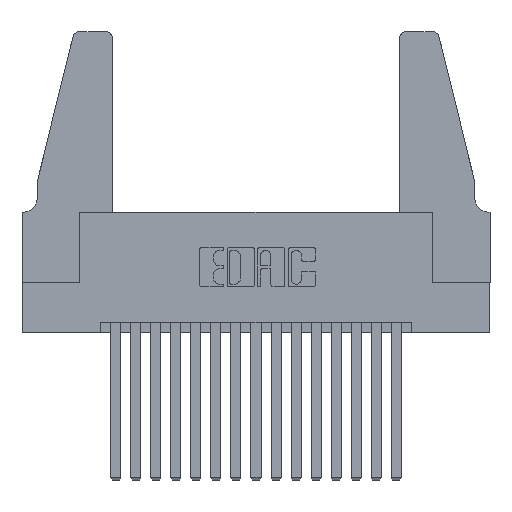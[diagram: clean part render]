
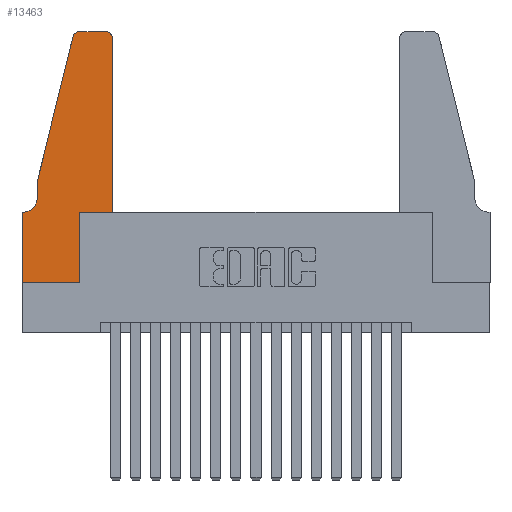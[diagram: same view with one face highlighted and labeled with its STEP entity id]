
A CAD part, top view. The second image highlights one B-rep face of the part: STEP entity #13463.
In plain terms, the highlighted planar face has unit normal (0, 0, 1).
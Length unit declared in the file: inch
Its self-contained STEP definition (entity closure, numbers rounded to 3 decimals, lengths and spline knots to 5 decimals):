
#137 = CARTESIAN_POINT ( 'NONE',  ( 0.284, 1.22, 0.37 ) ) ;
#166 = ORIENTED_EDGE ( 'NONE', *, *, #4814, .T. ) ;
#209 = LINE ( 'NONE', #13589, #14076 ) ;
#366 = DIRECTION ( 'NONE',  ( 0., 0., -1. ) ) ;
#385 = ORIENTED_EDGE ( 'NONE', *, *, #17398, .T. ) ;
#788 = CIRCLE ( 'NONE', #13161, 0.07 ) ;
#1159 = VECTOR ( 'NONE', #3147, 39.37008 ) ;
#1178 = EDGE_CURVE ( 'NONE', #5568, #14867, #12893, .T. ) ;
#1228 = EDGE_CURVE ( 'NONE', #10429, #8796, #16892, .T. ) ;
#1312 = EDGE_CURVE ( 'NONE', #3085, #3375, #16051, .T. ) ;
#1481 = DIRECTION ( 'NONE',  ( 1., 0., 0. ) ) ;
#1575 = DIRECTION ( 'NONE',  ( 0., 0., 1. ) ) ;
#1823 = DIRECTION ( 'NONE',  ( 0., 1., 0. ) ) ;
#1984 = CARTESIAN_POINT ( 'NONE',  ( 0.4205, 1.25, 0.37 ) ) ;
#2202 = CARTESIAN_POINT ( 'NONE',  ( 0.0755, 0.42, 0.37 ) ) ;
#2214 = LINE ( 'NONE', #5744, #1159 ) ;
#2564 = ORIENTED_EDGE ( 'NONE', *, *, #1178, .T. ) ;
#3085 = VERTEX_POINT ( 'NONE', #8862 ) ;
#3147 = DIRECTION ( 'NONE',  ( 1., 0., 0. ) ) ;
#3240 = CARTESIAN_POINT ( 'NONE',  ( 0.2605, 1.25, 0.37 ) ) ;
#3375 = VERTEX_POINT ( 'NONE', #8194 ) ;
#3391 = EDGE_CURVE ( 'NONE', #10705, #13900, #209, .T. ) ;
#3474 = CARTESIAN_POINT ( 'NONE',  ( 0.2865, 0.35, 0.37 ) ) ;
#3906 = CARTESIAN_POINT ( 'NONE',  ( 0.0055, 0.42, 0.37 ) ) ;
#3923 = FACE_OUTER_BOUND ( 'NONE', #4891, .T. ) ;
#3956 = LINE ( 'NONE', #12894, #6268 ) ;
#4252 = CARTESIAN_POINT ( 'NONE',  ( 0.4505, 0.35, 0.37 ) ) ;
#4470 = PLANE ( 'NONE',  #17057 ) ;
#4814 = EDGE_CURVE ( 'NONE', #3375, #9165, #5978, .T. ) ;
#4873 = VECTOR ( 'NONE', #11289, 39.37008 ) ;
#4891 = EDGE_LOOP ( 'NONE', ( #16648, #14484, #16259, #6245, #11322, #14737, #166, #10892, #2564, #385, #16778, #10352 ) ) ;
#5568 = VERTEX_POINT ( 'NONE', #9376 ) ;
#5744 = CARTESIAN_POINT ( 'NONE',  ( 0.4505, 0.35, 0.37 ) ) ;
#5761 = CARTESIAN_POINT ( 'NONE',  ( 0.4205, 1.22, 0.37 ) ) ;
#5942 = DIRECTION ( 'NONE',  ( -1., 0., 0. ) ) ;
#5945 = CARTESIAN_POINT ( 'NONE',  ( 0., 0., 0.37 ) ) ;
#5965 = VECTOR ( 'NONE', #1823, 39.37008 ) ;
#5978 = LINE ( 'NONE', #9507, #14577 ) ;
#6245 = ORIENTED_EDGE ( 'NONE', *, *, #8325, .T. ) ;
#6268 = VECTOR ( 'NONE', #16893, 39.37008 ) ;
#6347 = LINE ( 'NONE', #5945, #4873 ) ;
#6402 = CARTESIAN_POINT ( 'NONE',  ( 0.0755, 0.35, 0.37 ) ) ;
#6972 = EDGE_CURVE ( 'NONE', #10090, #10808, #15559, .T. ) ;
#7097 = CIRCLE ( 'NONE', #11618, 0.03 ) ;
#7509 = CARTESIAN_POINT ( 'NONE',  ( 0., 0., 0.37 ) ) ;
#7788 = CIRCLE ( 'NONE', #16339, 0.03 ) ;
#8117 = EDGE_CURVE ( 'NONE', #8409, #3085, #788, .T. ) ;
#8194 = CARTESIAN_POINT ( 'NONE',  ( 0., 0.35, 0.37 ) ) ;
#8314 = DIRECTION ( 'NONE',  ( 0., -1., 0. ) ) ;
#8325 = EDGE_CURVE ( 'NONE', #13900, #8409, #3956, .T. ) ;
#8409 = VERTEX_POINT ( 'NONE', #2202 ) ;
#8594 = DIRECTION ( 'NONE',  ( 0., 0., 1. ) ) ;
#8648 = CARTESIAN_POINT ( 'NONE',  ( 0., 0.35, 0.37 ) ) ;
#8796 = VERTEX_POINT ( 'NONE', #14611 ) ;
#8862 = CARTESIAN_POINT ( 'NONE',  ( 0.0055, 0.35, 0.37 ) ) ;
#9165 = VERTEX_POINT ( 'NONE', #7509 ) ;
#9376 = CARTESIAN_POINT ( 'NONE',  ( 0.2865, 0., 0.37 ) ) ;
#9507 = CARTESIAN_POINT ( 'NONE',  ( 0., 0., 0.37 ) ) ;
#9562 = DIRECTION ( 'NONE',  ( 0., 0., 1. ) ) ;
#10090 = VERTEX_POINT ( 'NONE', #13851 ) ;
#10174 = DIRECTION ( 'NONE',  ( -1., 0., 0. ) ) ;
#10352 = ORIENTED_EDGE ( 'NONE', *, *, #16832, .T. ) ;
#10429 = VERTEX_POINT ( 'NONE', #1984 ) ;
#10705 = VERTEX_POINT ( 'NONE', #12749 ) ;
#10747 = EDGE_CURVE ( 'NONE', #9165, #5568, #6347, .T. ) ;
#10808 = VERTEX_POINT ( 'NONE', #12856 ) ;
#10892 = ORIENTED_EDGE ( 'NONE', *, *, #10747, .T. ) ;
#10975 = DIRECTION ( 'NONE',  ( 1., 0., 0. ) ) ;
#11079 = CARTESIAN_POINT ( 'NONE',  ( 0.0755, 0.5, 0.37 ) ) ;
#11146 = VECTOR ( 'NONE', #16391, 39.37008 ) ;
#11289 = DIRECTION ( 'NONE',  ( 1., 0., 0. ) ) ;
#11322 = ORIENTED_EDGE ( 'NONE', *, *, #8117, .T. ) ;
#11618 = AXIS2_PLACEMENT_3D ( 'NONE', #5761, #1575, #10975 ) ;
#12103 = EDGE_CURVE ( 'NONE', #8796, #10705, #7788, .T. ) ;
#12272 = CARTESIAN_POINT ( 'NONE',  ( 0.2865, 0.35, 0.37 ) ) ;
#12619 = DIRECTION ( 'NONE',  ( 1., 0., 0. ) ) ;
#12681 = VECTOR ( 'NONE', #5942, 39.37008 ) ;
#12749 = CARTESIAN_POINT ( 'NONE',  ( 0.25487, 1.22718, 0.37 ) ) ;
#12856 = CARTESIAN_POINT ( 'NONE',  ( 0.4505, 1.22, 0.37 ) ) ;
#12893 = LINE ( 'NONE', #12272, #5965 ) ;
#12894 = CARTESIAN_POINT ( 'NONE',  ( 0.0755, 0.5, 0.37 ) ) ;
#13161 = AXIS2_PLACEMENT_3D ( 'NONE', #3906, #366, #13826 ) ;
#13463 = ADVANCED_FACE ( 'NONE', ( #3923 ), #4470, .T. ) ;
#13589 = CARTESIAN_POINT ( 'NONE',  ( 0.0755, 0.5, 0.37 ) ) ;
#13826 = DIRECTION ( 'NONE',  ( -1., 0., 0. ) ) ;
#13851 = CARTESIAN_POINT ( 'NONE',  ( 0.4505, 0.35, 0.37 ) ) ;
#13900 = VERTEX_POINT ( 'NONE', #11079 ) ;
#14076 = VECTOR ( 'NONE', #16118, 39.37008 ) ;
#14484 = ORIENTED_EDGE ( 'NONE', *, *, #12103, .T. ) ;
#14577 = VECTOR ( 'NONE', #8314, 39.37008 ) ;
#14611 = CARTESIAN_POINT ( 'NONE',  ( 0.284, 1.25, 0.37 ) ) ;
#14737 = ORIENTED_EDGE ( 'NONE', *, *, #1312, .T. ) ;
#14867 = VERTEX_POINT ( 'NONE', #3474 ) ;
#15559 = LINE ( 'NONE', #4252, #11146 ) ;
#16051 = LINE ( 'NONE', #6402, #16247 ) ;
#16118 = DIRECTION ( 'NONE',  ( -0.239, -0.971, 0. ) ) ;
#16247 = VECTOR ( 'NONE', #10174, 39.37008 ) ;
#16259 = ORIENTED_EDGE ( 'NONE', *, *, #3391, .T. ) ;
#16339 = AXIS2_PLACEMENT_3D ( 'NONE', #137, #9562, #1481 ) ;
#16391 = DIRECTION ( 'NONE',  ( 0., 1., 0. ) ) ;
#16648 = ORIENTED_EDGE ( 'NONE', *, *, #1228, .T. ) ;
#16778 = ORIENTED_EDGE ( 'NONE', *, *, #6972, .T. ) ;
#16832 = EDGE_CURVE ( 'NONE', #10808, #10429, #7097, .T. ) ;
#16892 = LINE ( 'NONE', #3240, #12681 ) ;
#16893 = DIRECTION ( 'NONE',  ( 0., -1., 0. ) ) ;
#17057 = AXIS2_PLACEMENT_3D ( 'NONE', #8648, #8594, #12619 ) ;
#17398 = EDGE_CURVE ( 'NONE', #14867, #10090, #2214, .T. ) ;
